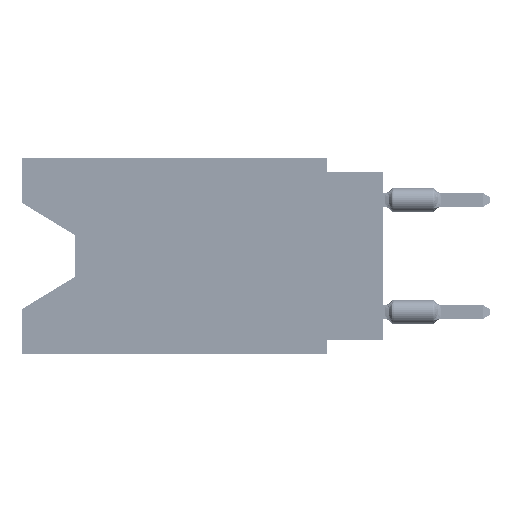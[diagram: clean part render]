
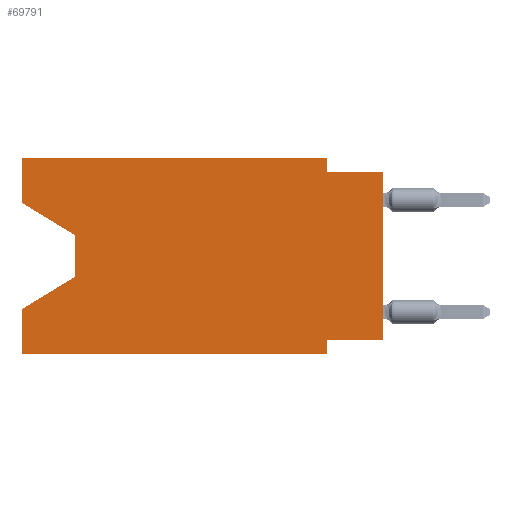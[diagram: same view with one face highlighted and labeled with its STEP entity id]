
A CAD part, left-side view. The second image highlights one B-rep face of the part: STEP entity #69791.
In plain terms, the highlighted planar face has unit normal (-1, 0, 0).
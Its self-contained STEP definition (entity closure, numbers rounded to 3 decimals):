
#759 = EDGE_CURVE ( 'NONE', #14384, #41255, #79655, .T. ) ;
#2409 = DIRECTION ( 'NONE',  ( 0., 1., 0. ) ) ;
#3002 = DIRECTION ( 'NONE',  ( 0., 0., -1. ) ) ;
#3878 = CARTESIAN_POINT ( 'NONE',  ( 0., 16.383, -2.038 ) ) ;
#6118 = VERTEX_POINT ( 'NONE', #16250 ) ;
#6279 = VECTOR ( 'NONE', #52458, 1000. ) ;
#6702 = DIRECTION ( 'NONE',  ( 0., -1., 0. ) ) ;
#6846 = EDGE_CURVE ( 'NONE', #90168, #47002, #13392, .T. ) ;
#9348 = CARTESIAN_POINT ( 'NONE',  ( 0., 16.383, 0. ) ) ;
#10845 = CARTESIAN_POINT ( 'NONE',  ( 0., 2.54, -0.635 ) ) ;
#11933 = EDGE_CURVE ( 'NONE', #90168, #67295, #99359, .T. ) ;
#12924 = CARTESIAN_POINT ( 'NONE',  ( 0., 13.97, -3.505 ) ) ;
#13288 = ORIENTED_EDGE ( 'NONE', *, *, #36034, .F. ) ;
#13392 = LINE ( 'NONE', #92861, #97426 ) ;
#13463 = EDGE_CURVE ( 'NONE', #66307, #69038, #23022, .T. ) ;
#14384 = VERTEX_POINT ( 'NONE', #9348 ) ;
#15012 = CARTESIAN_POINT ( 'NONE',  ( 0., 16.383, 0. ) ) ;
#16250 = CARTESIAN_POINT ( 'NONE',  ( 0., 2.54, -8.89 ) ) ;
#17975 = VECTOR ( 'NONE', #77704, 1000. ) ;
#18199 = EDGE_CURVE ( 'NONE', #55440, #42117, #20147, .T. ) ;
#18467 = DIRECTION ( 'NONE',  ( 0., -1., 0. ) ) ;
#19950 = DIRECTION ( 'NONE',  ( 0., 0., -1. ) ) ;
#20147 = LINE ( 'NONE', #23161, #6279 ) ;
#20937 = CARTESIAN_POINT ( 'NONE',  ( 0., 0., -0.635 ) ) ;
#21744 = ORIENTED_EDGE ( 'NONE', *, *, #62535, .F. ) ;
#22613 = LINE ( 'NONE', #55450, #41681 ) ;
#23022 = LINE ( 'NONE', #79195, #78427 ) ;
#23161 = CARTESIAN_POINT ( 'NONE',  ( 0., 13.97, -5.385 ) ) ;
#23891 = CARTESIAN_POINT ( 'NONE',  ( 0., 0., -8.255 ) ) ;
#26258 = CARTESIAN_POINT ( 'NONE',  ( 0., 0., -8.255 ) ) ;
#27888 = LINE ( 'NONE', #59697, #94499 ) ;
#28604 = EDGE_CURVE ( 'NONE', #48198, #42117, #77454, .T. ) ;
#30762 = ORIENTED_EDGE ( 'NONE', *, *, #6846, .T. ) ;
#32260 = ORIENTED_EDGE ( 'NONE', *, *, #59900, .T. ) ;
#35562 = LINE ( 'NONE', #36612, #39036 ) ;
#36034 = EDGE_CURVE ( 'NONE', #58620, #47002, #22613, .T. ) ;
#36612 = CARTESIAN_POINT ( 'NONE',  ( 0., 16.383, 0. ) ) ;
#37509 = CARTESIAN_POINT ( 'NONE',  ( 0., 2.54, 0. ) ) ;
#39036 = VECTOR ( 'NONE', #68451, 1000. ) ;
#39046 = ORIENTED_EDGE ( 'NONE', *, *, #18199, .T. ) ;
#39659 = AXIS2_PLACEMENT_3D ( 'NONE', #51751, #66106, #3002 ) ;
#40333 = VECTOR ( 'NONE', #2409, 1000. ) ;
#41255 = VERTEX_POINT ( 'NONE', #71360 ) ;
#41681 = VECTOR ( 'NONE', #6702, 1000. ) ;
#42117 = VERTEX_POINT ( 'NONE', #102898 ) ;
#42228 = FACE_OUTER_BOUND ( 'NONE', #62300, .T. ) ;
#43329 = CARTESIAN_POINT ( 'NONE',  ( 0., 16.383, -8.89 ) ) ;
#43392 = CARTESIAN_POINT ( 'NONE',  ( 0., 13.97, -5.385 ) ) ;
#47002 = VERTEX_POINT ( 'NONE', #20937 ) ;
#48198 = VERTEX_POINT ( 'NONE', #56144 ) ;
#48374 = EDGE_CURVE ( 'NONE', #48198, #6118, #100564, .T. ) ;
#51525 = EDGE_CURVE ( 'NONE', #67295, #6118, #99570, .T. ) ;
#51751 = CARTESIAN_POINT ( 'NONE',  ( 0., 16.383, 0. ) ) ;
#52458 = DIRECTION ( 'NONE',  ( 0., 0.855, -0.519 ) ) ;
#53427 = LINE ( 'NONE', #37509, #81552 ) ;
#53772 = ORIENTED_EDGE ( 'NONE', *, *, #81413, .F. ) ;
#55440 = VERTEX_POINT ( 'NONE', #43392 ) ;
#55450 = CARTESIAN_POINT ( 'NONE',  ( 0., 0., -0.635 ) ) ;
#55757 = ORIENTED_EDGE ( 'NONE', *, *, #11933, .F. ) ;
#55799 = DIRECTION ( 'NONE',  ( 0., -1., 0. ) ) ;
#55868 = VECTOR ( 'NONE', #55799, 1000. ) ;
#56144 = CARTESIAN_POINT ( 'NONE',  ( 0., 16.383, -8.89 ) ) ;
#57084 = ORIENTED_EDGE ( 'NONE', *, *, #759, .F. ) ;
#58620 = VERTEX_POINT ( 'NONE', #10845 ) ;
#59697 = CARTESIAN_POINT ( 'NONE',  ( 0., 13.97, -3.505 ) ) ;
#59900 = EDGE_CURVE ( 'NONE', #69038, #55440, #27888, .T. ) ;
#60494 = CARTESIAN_POINT ( 'NONE',  ( 0., 16.383, 0. ) ) ;
#62300 = EDGE_LOOP ( 'NONE', ( #82760, #32260, #39046, #76351, #97473, #77518, #55757, #30762, #13288, #53772, #57084, #21744 ) ) ;
#62535 = EDGE_CURVE ( 'NONE', #66307, #14384, #35562, .T. ) ;
#66106 = DIRECTION ( 'NONE',  ( 1., 0., 0. ) ) ;
#66307 = VERTEX_POINT ( 'NONE', #3878 ) ;
#66627 = PLANE ( 'NONE',  #39659 ) ;
#67295 = VERTEX_POINT ( 'NONE', #76693 ) ;
#68451 = DIRECTION ( 'NONE',  ( 0., 0., 1. ) ) ;
#69038 = VERTEX_POINT ( 'NONE', #12924 ) ;
#69791 = ADVANCED_FACE ( 'NONE', ( #42228 ), #66627, .F. ) ;
#71360 = CARTESIAN_POINT ( 'NONE',  ( 0., 2.54, 0. ) ) ;
#74708 = CARTESIAN_POINT ( 'NONE',  ( 0., 2.54, -8.89 ) ) ;
#76351 = ORIENTED_EDGE ( 'NONE', *, *, #28604, .F. ) ;
#76693 = CARTESIAN_POINT ( 'NONE',  ( 0., 2.54, -8.255 ) ) ;
#77454 = LINE ( 'NONE', #60494, #91459 ) ;
#77518 = ORIENTED_EDGE ( 'NONE', *, *, #51525, .F. ) ;
#77704 = DIRECTION ( 'NONE',  ( 0., 0., -1. ) ) ;
#78427 = VECTOR ( 'NONE', #104092, 1000. ) ;
#79195 = CARTESIAN_POINT ( 'NONE',  ( 0., 16.383, -2.038 ) ) ;
#79655 = LINE ( 'NONE', #15012, #55868 ) ;
#81413 = EDGE_CURVE ( 'NONE', #41255, #58620, #53427, .T. ) ;
#81552 = VECTOR ( 'NONE', #85755, 1000. ) ;
#82760 = ORIENTED_EDGE ( 'NONE', *, *, #13463, .T. ) ;
#85402 = DIRECTION ( 'NONE',  ( 0., 0., 1. ) ) ;
#85453 = DIRECTION ( 'NONE',  ( 0., 0., 1. ) ) ;
#85755 = DIRECTION ( 'NONE',  ( 0., 0., -1. ) ) ;
#90168 = VERTEX_POINT ( 'NONE', #23891 ) ;
#90334 = VECTOR ( 'NONE', #18467, 1000. ) ;
#91459 = VECTOR ( 'NONE', #85402, 1000. ) ;
#92861 = CARTESIAN_POINT ( 'NONE',  ( 0., 0., 0. ) ) ;
#94499 = VECTOR ( 'NONE', #19950, 1000. ) ;
#97426 = VECTOR ( 'NONE', #85453, 1000. ) ;
#97473 = ORIENTED_EDGE ( 'NONE', *, *, #48374, .T. ) ;
#99359 = LINE ( 'NONE', #26258, #40333 ) ;
#99570 = LINE ( 'NONE', #74708, #17975 ) ;
#100564 = LINE ( 'NONE', #43329, #90334 ) ;
#102898 = CARTESIAN_POINT ( 'NONE',  ( 0., 16.383, -6.852 ) ) ;
#104092 = DIRECTION ( 'NONE',  ( 0., -0.855, -0.519 ) ) ;
